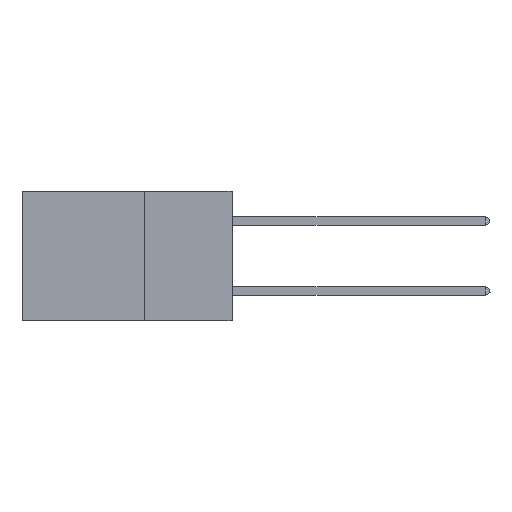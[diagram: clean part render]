
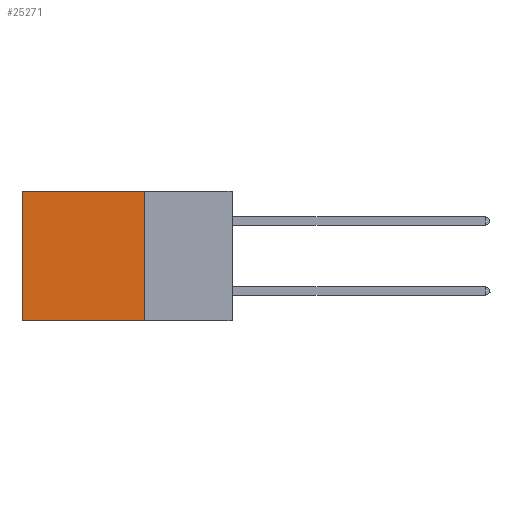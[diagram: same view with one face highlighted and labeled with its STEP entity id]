
A CAD part, left-side view. The second image highlights one B-rep face of the part: STEP entity #25271.
In plain terms, the highlighted planar face has unit normal (-1, 0, 0).
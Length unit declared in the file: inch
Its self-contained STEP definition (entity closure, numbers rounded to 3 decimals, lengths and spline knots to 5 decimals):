
#214 = CARTESIAN_POINT ( 'NONE',  ( 0.2875, 0.6, 0. ) ) ;
#572 = VERTEX_POINT ( 'NONE', #25230 ) ;
#1169 = CARTESIAN_POINT ( 'NONE',  ( 0.2875, 0.25, -0.37 ) ) ;
#2178 = VECTOR ( 'NONE', #13900, 39.37008 ) ;
#2335 = EDGE_CURVE ( 'NONE', #10494, #20061, #20110, .T. ) ;
#2338 = DIRECTION ( 'NONE',  ( 0., 0., -1. ) ) ;
#2905 = LINE ( 'NONE', #9858, #9695 ) ;
#4745 = VERTEX_POINT ( 'NONE', #6826 ) ;
#5135 = EDGE_CURVE ( 'NONE', #4745, #572, #12495, .T. ) ;
#6826 = CARTESIAN_POINT ( 'NONE',  ( 0.2875, 0.6, 0. ) ) ;
#7367 = EDGE_CURVE ( 'NONE', #10494, #4745, #2905, .T. ) ;
#9695 = VECTOR ( 'NONE', #26575, 39.37008 ) ;
#9858 = CARTESIAN_POINT ( 'NONE',  ( 0.2875, 0.25, 0. ) ) ;
#9921 = CARTESIAN_POINT ( 'NONE',  ( 0.2875, 0.25, 0. ) ) ;
#10494 = VERTEX_POINT ( 'NONE', #13033 ) ;
#12495 = LINE ( 'NONE', #214, #19360 ) ;
#13033 = CARTESIAN_POINT ( 'NONE',  ( 0.2875, 0.25, 0. ) ) ;
#13160 = EDGE_CURVE ( 'NONE', #20061, #572, #18804, .T. ) ;
#13441 = ORIENTED_EDGE ( 'NONE', *, *, #7367, .T. ) ;
#13900 = DIRECTION ( 'NONE',  ( 0., 1., 0. ) ) ;
#14217 = PLANE ( 'NONE',  #16310 ) ;
#14602 = ORIENTED_EDGE ( 'NONE', *, *, #13160, .F. ) ;
#16310 = AXIS2_PLACEMENT_3D ( 'NONE', #9921, #22371, #24469 ) ;
#16762 = CARTESIAN_POINT ( 'NONE',  ( 0.2875, 0.25, 0. ) ) ;
#17531 = ORIENTED_EDGE ( 'NONE', *, *, #2335, .F. ) ;
#18804 = LINE ( 'NONE', #1169, #2178 ) ;
#18871 = DIRECTION ( 'NONE',  ( 0., 0., -1. ) ) ;
#19360 = VECTOR ( 'NONE', #2338, 39.37008 ) ;
#20061 = VERTEX_POINT ( 'NONE', #25716 ) ;
#20110 = LINE ( 'NONE', #16762, #24039 ) ;
#21711 = EDGE_LOOP ( 'NONE', ( #24149, #14602, #17531, #13441 ) ) ;
#22371 = DIRECTION ( 'NONE',  ( 1., 0., 0. ) ) ;
#23859 = FACE_OUTER_BOUND ( 'NONE', #21711, .T. ) ;
#24039 = VECTOR ( 'NONE', #18871, 39.37008 ) ;
#24149 = ORIENTED_EDGE ( 'NONE', *, *, #5135, .T. ) ;
#24469 = DIRECTION ( 'NONE',  ( 0., 0., -1. ) ) ;
#25230 = CARTESIAN_POINT ( 'NONE',  ( 0.2875, 0.6, -0.37 ) ) ;
#25271 = ADVANCED_FACE ( 'NONE', ( #23859 ), #14217, .F. ) ;
#25716 = CARTESIAN_POINT ( 'NONE',  ( 0.2875, 0.25, -0.37 ) ) ;
#26575 = DIRECTION ( 'NONE',  ( 0., 1., 0. ) ) ;
